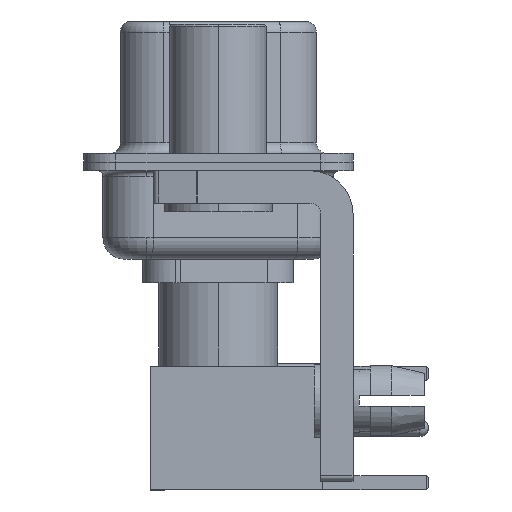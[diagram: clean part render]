
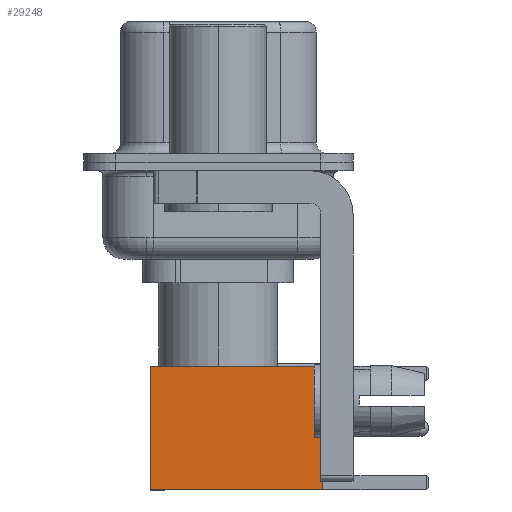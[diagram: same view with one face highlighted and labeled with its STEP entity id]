
A CAD part, left-side view. The second image highlights one B-rep face of the part: STEP entity #29248.
In plain terms, the highlighted face is planar.
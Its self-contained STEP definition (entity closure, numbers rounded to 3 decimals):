
#1663 = DIRECTION ( 'NONE',  ( 0., 0., -1. ) ) ;
#2041 = CARTESIAN_POINT ( 'NONE',  ( 2.875, 2.875, 0. ) ) ;
#2326 = FACE_OUTER_BOUND ( 'NONE', #18125, .T. ) ;
#2864 = DIRECTION ( 'NONE',  ( -1., 0., 0. ) ) ;
#4109 = DIRECTION ( 'NONE',  ( 0., 0., -1. ) ) ;
#4280 = LINE ( 'NONE', #33365, #18195 ) ;
#4874 = ORIENTED_EDGE ( 'NONE', *, *, #20090, .T. ) ;
#4944 = CARTESIAN_POINT ( 'NONE',  ( 2.875, 2.875, 0. ) ) ;
#6719 = CARTESIAN_POINT ( 'NONE',  ( 2.875, 2.875, 0. ) ) ;
#6768 = LINE ( 'NONE', #20193, #24972 ) ;
#7402 = VERTEX_POINT ( 'NONE', #2041 ) ;
#10375 = DIRECTION ( 'NONE',  ( 0., 1., 0. ) ) ;
#11261 = CARTESIAN_POINT ( 'NONE',  ( -2.875, 2.875, 8. ) ) ;
#11605 = EDGE_CURVE ( 'NONE', #31998, #32204, #4280, .T. ) ;
#11656 = VECTOR ( 'NONE', #2864, 1000. ) ;
#12897 = ORIENTED_EDGE ( 'NONE', *, *, #17737, .F. ) ;
#13797 = PLANE ( 'NONE',  #32117 ) ;
#15607 = CARTESIAN_POINT ( 'NONE',  ( -2.875, 2.875, 0. ) ) ;
#15762 = VERTEX_POINT ( 'NONE', #34342 ) ;
#16035 = ORIENTED_EDGE ( 'NONE', *, *, #11605, .F. ) ;
#16906 = EDGE_CURVE ( 'NONE', #7402, #32204, #6768, .T. ) ;
#17737 = EDGE_CURVE ( 'NONE', #15762, #31998, #29696, .T. ) ;
#18125 = EDGE_LOOP ( 'NONE', ( #4874, #32158, #16035, #12897 ) ) ;
#18195 = VECTOR ( 'NONE', #4109, 1000. ) ;
#19964 = LINE ( 'NONE', #6719, #32885 ) ;
#20090 = EDGE_CURVE ( 'NONE', #15762, #7402, #19964, .T. ) ;
#20193 = CARTESIAN_POINT ( 'NONE',  ( 0., 2.875, 0. ) ) ;
#24972 = VECTOR ( 'NONE', #28032, 1000. ) ;
#26759 = CARTESIAN_POINT ( 'NONE',  ( 0., 2.875, 8. ) ) ;
#28032 = DIRECTION ( 'NONE',  ( -1., 0., 0. ) ) ;
#28809 = DIRECTION ( 'NONE',  ( 0., 0., 1. ) ) ;
#29248 = ADVANCED_FACE ( 'NONE', ( #2326 ), #13797, .T. ) ;
#29696 = LINE ( 'NONE', #26759, #11656 ) ;
#31998 = VERTEX_POINT ( 'NONE', #11261 ) ;
#32117 = AXIS2_PLACEMENT_3D ( 'NONE', #4944, #10375, #28809 ) ;
#32158 = ORIENTED_EDGE ( 'NONE', *, *, #16906, .T. ) ;
#32204 = VERTEX_POINT ( 'NONE', #15607 ) ;
#32885 = VECTOR ( 'NONE', #1663, 1000. ) ;
#33365 = CARTESIAN_POINT ( 'NONE',  ( -2.875, 2.875, 0. ) ) ;
#34342 = CARTESIAN_POINT ( 'NONE',  ( 2.875, 2.875, 8. ) ) ;
